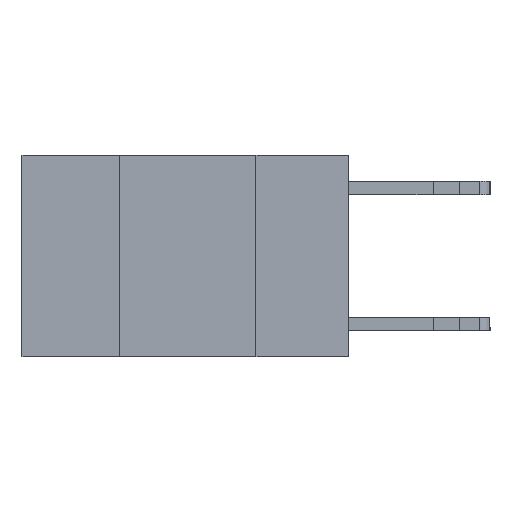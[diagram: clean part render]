
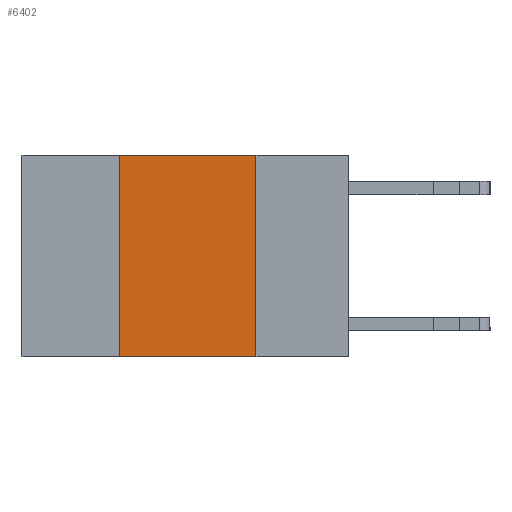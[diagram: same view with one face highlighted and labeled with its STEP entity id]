
A CAD part, left-side view. The second image highlights one B-rep face of the part: STEP entity #6402.
In plain terms, the highlighted planar face has unit normal (-1, 0, 0).
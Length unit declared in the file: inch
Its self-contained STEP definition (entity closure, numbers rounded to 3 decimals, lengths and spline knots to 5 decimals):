
#1634 = DIRECTION ( 'NONE',  ( 0., 0., -1. ) ) ;
#1787 = CARTESIAN_POINT ( 'NONE',  ( 0., 0.42, 0. ) ) ;
#2009 = VERTEX_POINT ( 'NONE', #5435 ) ;
#2126 = VECTOR ( 'NONE', #8787, 39.37008 ) ;
#2499 = VERTEX_POINT ( 'NONE', #3118 ) ;
#2674 = CARTESIAN_POINT ( 'NONE',  ( 0., 0.42, -0.37 ) ) ;
#2790 = EDGE_CURVE ( 'NONE', #2009, #2499, #4164, .T. ) ;
#3111 = DIRECTION ( 'NONE',  ( 0., -1., 0. ) ) ;
#3118 = CARTESIAN_POINT ( 'NONE',  ( 0., 0.17, -0.37 ) ) ;
#3735 = DIRECTION ( 'NONE',  ( 0., -1., 0. ) ) ;
#3847 = CARTESIAN_POINT ( 'NONE',  ( 0., 0.6, 0. ) ) ;
#4016 = DIRECTION ( 'NONE',  ( 1., 0., 0. ) ) ;
#4083 = CARTESIAN_POINT ( 'NONE',  ( 0., 0.17, 0. ) ) ;
#4164 = LINE ( 'NONE', #4083, #2126 ) ;
#4343 = CARTESIAN_POINT ( 'NONE',  ( 0., 0.6, -0.37 ) ) ;
#4574 = VECTOR ( 'NONE', #3111, 39.37008 ) ;
#5026 = CARTESIAN_POINT ( 'NONE',  ( 0., 0.6, 0. ) ) ;
#5435 = CARTESIAN_POINT ( 'NONE',  ( 0., 0.17, 0. ) ) ;
#5543 = DIRECTION ( 'NONE',  ( 0., 0., 1. ) ) ;
#5655 = VERTEX_POINT ( 'NONE', #11382 ) ;
#6402 = ADVANCED_FACE ( 'NONE', ( #11499 ), #8784, .F. ) ;
#6521 = ORIENTED_EDGE ( 'NONE', *, *, #7392, .F. ) ;
#6649 = EDGE_CURVE ( 'NONE', #10964, #5655, #7893, .T. ) ;
#6759 = EDGE_LOOP ( 'NONE', ( #8179, #6521, #12961, #14052 ) ) ;
#7392 = EDGE_CURVE ( 'NONE', #5655, #2009, #10048, .T. ) ;
#7615 = AXIS2_PLACEMENT_3D ( 'NONE', #3847, #4016, #1634 ) ;
#7893 = LINE ( 'NONE', #1787, #15193 ) ;
#8179 = ORIENTED_EDGE ( 'NONE', *, *, #2790, .F. ) ;
#8784 = PLANE ( 'NONE',  #7615 ) ;
#8787 = DIRECTION ( 'NONE',  ( 0., 0., -1. ) ) ;
#9280 = LINE ( 'NONE', #4343, #4574 ) ;
#10048 = LINE ( 'NONE', #5026, #11020 ) ;
#10352 = EDGE_CURVE ( 'NONE', #10964, #2499, #9280, .T. ) ;
#10964 = VERTEX_POINT ( 'NONE', #2674 ) ;
#11020 = VECTOR ( 'NONE', #3735, 39.37008 ) ;
#11382 = CARTESIAN_POINT ( 'NONE',  ( 0., 0.42, 0. ) ) ;
#11499 = FACE_OUTER_BOUND ( 'NONE', #6759, .T. ) ;
#12961 = ORIENTED_EDGE ( 'NONE', *, *, #6649, .F. ) ;
#14052 = ORIENTED_EDGE ( 'NONE', *, *, #10352, .T. ) ;
#15193 = VECTOR ( 'NONE', #5543, 39.37008 ) ;
